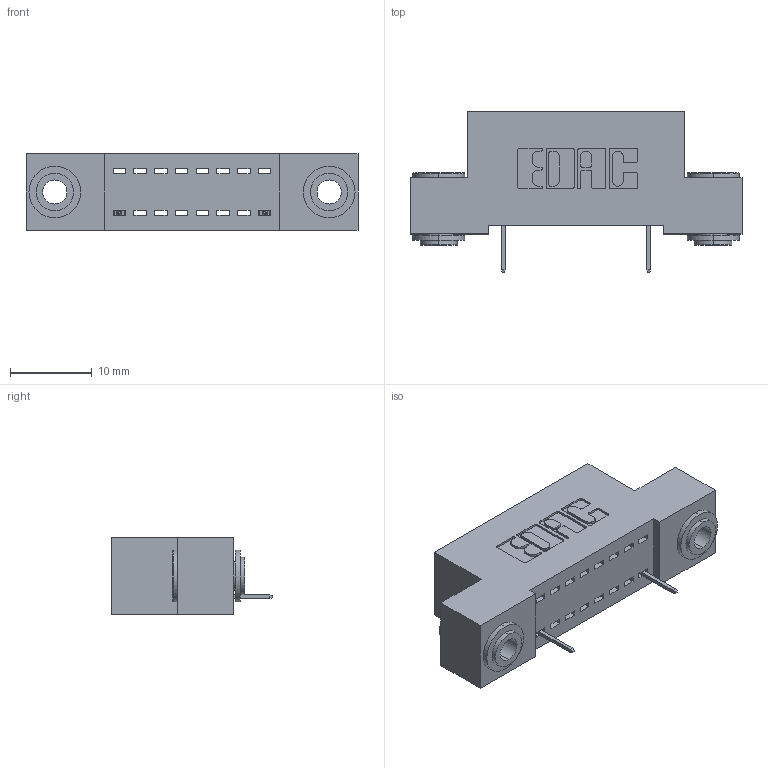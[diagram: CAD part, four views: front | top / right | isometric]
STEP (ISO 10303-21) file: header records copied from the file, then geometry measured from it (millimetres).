
FILE_DESCRIPTION (( 'STEP AP203' ), '1' );
FILE_NAME ('392-008-524-103.STEP', '2018-08-14T19:15:33', ( '' ), ( '' ), 'SwSTEP 2.0', 'SolidWorks 2016', '' );
FILE_SCHEMA (( 'CONFIG_CONTROL_DESIGN' ));
Length unit declared in the file: inch
Products named in the file (4): 342-250-002_345-250-002-102; 392-008-524-103; 342 Part_.156 TH; 345-292-001_345-293-124
Assembly tree (5 placements, depth 2):
  392-008-524-103
    342 Part_.156 TH
    345-292-001_345-293-124  x2
    342-250-002_345-250-002-102  x2
Bounding box: 40.64 x 19.69 x 9.4 mm (x, y, z)
Volume: 3384.4 mm3; surface area: 4181 mm2
Topology: 5 solids, 5 shells, 344 faces, 987 edges, 646 vertices
Faces by surface type: plane 244, cylinder 92, cone 8
Entity records: 9688 total; most frequent: CARTESIAN_POINT 1679, ORIENTED_EDGE 1622, DIRECTION 1513, EDGE_CURVE 811, LINE 663, VECTOR 663, VERTEX_POINT 534, AXIS2_PLACEMENT_3D 425
